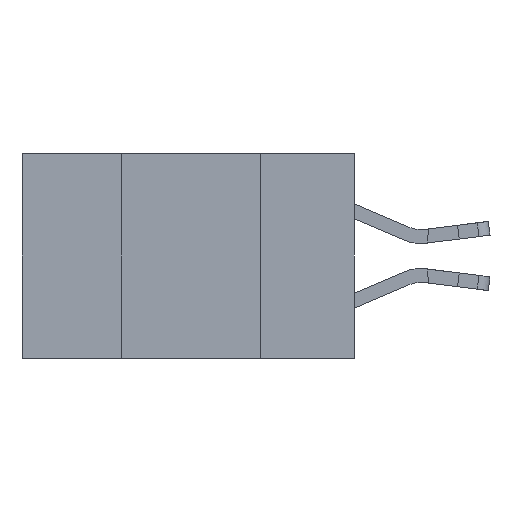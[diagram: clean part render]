
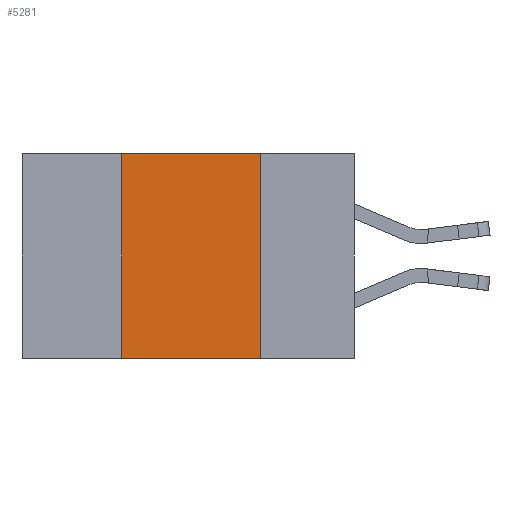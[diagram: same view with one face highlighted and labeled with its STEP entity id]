
A CAD part, left-side view. The second image highlights one B-rep face of the part: STEP entity #5281.
In plain terms, the highlighted planar face has unit normal (-1, 0, 0).
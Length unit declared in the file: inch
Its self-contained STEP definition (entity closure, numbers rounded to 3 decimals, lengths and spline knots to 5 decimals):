
#296 = LINE ( 'NONE', #14221, #6821 ) ;
#450 = VERTEX_POINT ( 'NONE', #902 ) ;
#538 = DIRECTION ( 'NONE',  ( 1., 0., 0. ) ) ;
#902 = CARTESIAN_POINT ( 'NONE',  ( 0., 0.17, -0.37 ) ) ;
#943 = EDGE_CURVE ( 'NONE', #3872, #450, #3137, .T. ) ;
#1085 = LINE ( 'NONE', #6167, #11939 ) ;
#2441 = CARTESIAN_POINT ( 'NONE',  ( 0., 0.42, 0. ) ) ;
#2672 = DIRECTION ( 'NONE',  ( 0., 0., -1. ) ) ;
#3054 = DIRECTION ( 'NONE',  ( 0., -1., 0. ) ) ;
#3137 = LINE ( 'NONE', #9435, #3813 ) ;
#3151 = DIRECTION ( 'NONE',  ( 0., 0., -1. ) ) ;
#3813 = VECTOR ( 'NONE', #3054, 39.37008 ) ;
#3868 = LINE ( 'NONE', #10279, #7133 ) ;
#3872 = VERTEX_POINT ( 'NONE', #16630 ) ;
#4934 = DIRECTION ( 'NONE',  ( 0., -1., 0. ) ) ;
#5281 = ADVANCED_FACE ( 'NONE', ( #10656 ), #10811, .F. ) ;
#6065 = CARTESIAN_POINT ( 'NONE',  ( 0., 0.17, 0. ) ) ;
#6167 = CARTESIAN_POINT ( 'NONE',  ( 0., 0.6, 0. ) ) ;
#6626 = VERTEX_POINT ( 'NONE', #2441 ) ;
#6821 = VECTOR ( 'NONE', #2672, 39.37008 ) ;
#7133 = VECTOR ( 'NONE', #14418, 39.37008 ) ;
#8101 = ORIENTED_EDGE ( 'NONE', *, *, #13637, .F. ) ;
#9002 = VERTEX_POINT ( 'NONE', #6065 ) ;
#9435 = CARTESIAN_POINT ( 'NONE',  ( 0., 0.6, -0.37 ) ) ;
#10278 = AXIS2_PLACEMENT_3D ( 'NONE', #12055, #538, #3151 ) ;
#10279 = CARTESIAN_POINT ( 'NONE',  ( 0., 0.42, -0.37 ) ) ;
#10656 = FACE_OUTER_BOUND ( 'NONE', #16365, .T. ) ;
#10811 = PLANE ( 'NONE',  #10278 ) ;
#11939 = VECTOR ( 'NONE', #4934, 39.37008 ) ;
#12055 = CARTESIAN_POINT ( 'NONE',  ( 0., 0.6, 0. ) ) ;
#13578 = ORIENTED_EDGE ( 'NONE', *, *, #13848, .F. ) ;
#13637 = EDGE_CURVE ( 'NONE', #6626, #9002, #1085, .T. ) ;
#13819 = ORIENTED_EDGE ( 'NONE', *, *, #14801, .F. ) ;
#13848 = EDGE_CURVE ( 'NONE', #9002, #450, #296, .T. ) ;
#14036 = ORIENTED_EDGE ( 'NONE', *, *, #943, .T. ) ;
#14221 = CARTESIAN_POINT ( 'NONE',  ( 0., 0.17, -0.37 ) ) ;
#14418 = DIRECTION ( 'NONE',  ( 0., 0., 1. ) ) ;
#14801 = EDGE_CURVE ( 'NONE', #3872, #6626, #3868, .T. ) ;
#16365 = EDGE_LOOP ( 'NONE', ( #13578, #8101, #13819, #14036 ) ) ;
#16630 = CARTESIAN_POINT ( 'NONE',  ( 0., 0.42, -0.37 ) ) ;
